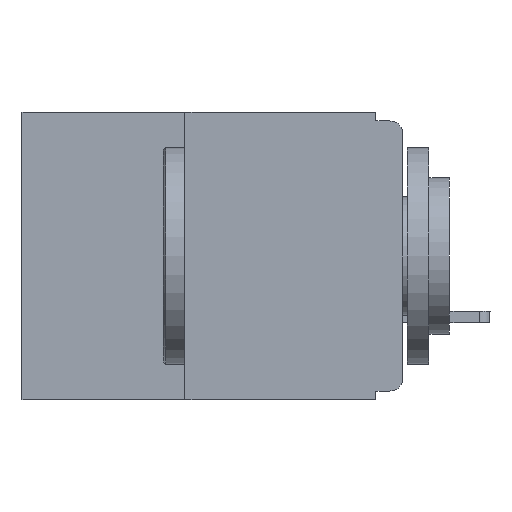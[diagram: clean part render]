
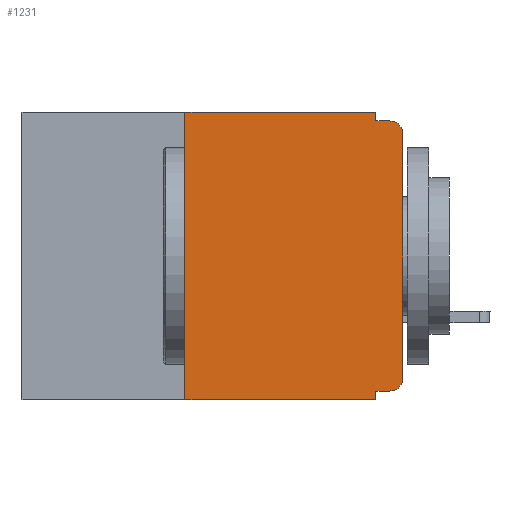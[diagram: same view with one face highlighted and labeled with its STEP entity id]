
A CAD part, left-side view. The second image highlights one B-rep face of the part: STEP entity #1231.
In plain terms, the highlighted planar face has unit normal (-1, 0, 0).
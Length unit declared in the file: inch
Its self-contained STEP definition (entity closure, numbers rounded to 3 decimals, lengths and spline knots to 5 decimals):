
#400 = CARTESIAN_POINT ( 'NONE',  ( 0., 0.015, -0.025 ) ) ;
#555 = CARTESIAN_POINT ( 'NONE',  ( 0., 0.25, -0.33 ) ) ;
#759 = CARTESIAN_POINT ( 'NONE',  ( 0., 0.031, -0.32 ) ) ;
#765 = CARTESIAN_POINT ( 'NONE',  ( 0., 0.25, -0.33 ) ) ;
#837 = AXIS2_PLACEMENT_3D ( 'NONE', #400, #8403, #2529 ) ;
#1047 = CARTESIAN_POINT ( 'NONE',  ( 0., 0.25, 0. ) ) ;
#1231 = ADVANCED_FACE ( 'NONE', ( #4734 ), #10816, .F. ) ;
#1257 = ORIENTED_EDGE ( 'NONE', *, *, #12819, .T. ) ;
#1426 = VERTEX_POINT ( 'NONE', #13756 ) ;
#1463 = LINE ( 'NONE', #3609, #4878 ) ;
#1474 = EDGE_CURVE ( 'NONE', #14251, #2308, #5824, .T. ) ;
#1595 = DIRECTION ( 'NONE',  ( 0., 1., 0. ) ) ;
#1704 = ORIENTED_EDGE ( 'NONE', *, *, #1474, .T. ) ;
#1735 = CARTESIAN_POINT ( 'NONE',  ( 0., 0., -0.01 ) ) ;
#1940 = EDGE_CURVE ( 'NONE', #13731, #7033, #12587, .T. ) ;
#2224 = CARTESIAN_POINT ( 'NONE',  ( 0., 0.015, -0.01 ) ) ;
#2284 = EDGE_CURVE ( 'NONE', #1426, #12051, #12751, .T. ) ;
#2308 = VERTEX_POINT ( 'NONE', #3808 ) ;
#2529 = DIRECTION ( 'NONE',  ( 0., 0., -1. ) ) ;
#2560 = ORIENTED_EDGE ( 'NONE', *, *, #7017, .F. ) ;
#2959 = VECTOR ( 'NONE', #10893, 39.37008 ) ;
#3289 = ORIENTED_EDGE ( 'NONE', *, *, #1940, .F. ) ;
#3340 = AXIS2_PLACEMENT_3D ( 'NONE', #14226, #7189, #14316 ) ;
#3463 = EDGE_CURVE ( 'NONE', #14881, #12051, #5784, .T. ) ;
#3609 = CARTESIAN_POINT ( 'NONE',  ( 0., 0., 0. ) ) ;
#3663 = DIRECTION ( 'NONE',  ( 0., 0., 1. ) ) ;
#3808 = CARTESIAN_POINT ( 'NONE',  ( 0., 0., -0.305 ) ) ;
#3840 = ORIENTED_EDGE ( 'NONE', *, *, #8504, .T. ) ;
#4064 = EDGE_CURVE ( 'NONE', #6564, #12901, #7020, .T. ) ;
#4211 = CARTESIAN_POINT ( 'NONE',  ( 0., 0.437, -0.33 ) ) ;
#4337 = CARTESIAN_POINT ( 'NONE',  ( 0., 0.031, 0. ) ) ;
#4423 = CARTESIAN_POINT ( 'NONE',  ( 0., 0.031, -0.33 ) ) ;
#4428 = ORIENTED_EDGE ( 'NONE', *, *, #13892, .F. ) ;
#4734 = FACE_OUTER_BOUND ( 'NONE', #10722, .T. ) ;
#4878 = VECTOR ( 'NONE', #3663, 39.37008 ) ;
#5418 = VECTOR ( 'NONE', #10131, 39.37008 ) ;
#5421 = DIRECTION ( 'NONE',  ( 0., -1., 0. ) ) ;
#5551 = CARTESIAN_POINT ( 'NONE',  ( 0., 0.015, -0.305 ) ) ;
#5646 = CARTESIAN_POINT ( 'NONE',  ( 0., 0.437, 0. ) ) ;
#5756 = LINE ( 'NONE', #5646, #6821 ) ;
#5784 = LINE ( 'NONE', #1735, #7935 ) ;
#5824 = CIRCLE ( 'NONE', #11111, 0.015 ) ;
#6564 = VERTEX_POINT ( 'NONE', #759 ) ;
#6794 = CARTESIAN_POINT ( 'NONE',  ( 0., 0.031, 0. ) ) ;
#6795 = DIRECTION ( 'NONE',  ( 0., -1., 0. ) ) ;
#6821 = VECTOR ( 'NONE', #6795, 39.37008 ) ;
#7017 = EDGE_CURVE ( 'NONE', #8080, #14881, #10068, .T. ) ;
#7020 = LINE ( 'NONE', #4423, #5418 ) ;
#7033 = VERTEX_POINT ( 'NONE', #1047 ) ;
#7097 = EDGE_CURVE ( 'NONE', #14251, #6564, #8948, .T. ) ;
#7189 = DIRECTION ( 'NONE',  ( 1., 0., 0. ) ) ;
#7916 = DIRECTION ( 'NONE',  ( 0., 0., -1. ) ) ;
#7935 = VECTOR ( 'NONE', #10973, 39.37008 ) ;
#8024 = ORIENTED_EDGE ( 'NONE', *, *, #7097, .F. ) ;
#8080 = VERTEX_POINT ( 'NONE', #6794 ) ;
#8403 = DIRECTION ( 'NONE',  ( -1., 0., 0. ) ) ;
#8426 = ORIENTED_EDGE ( 'NONE', *, *, #2284, .T. ) ;
#8504 = EDGE_CURVE ( 'NONE', #13731, #12901, #14131, .T. ) ;
#8948 = LINE ( 'NONE', #12123, #11563 ) ;
#9045 = DIRECTION ( 'NONE',  ( -1., 0., 0. ) ) ;
#9204 = ORIENTED_EDGE ( 'NONE', *, *, #4064, .F. ) ;
#10068 = LINE ( 'NONE', #4337, #11917 ) ;
#10131 = DIRECTION ( 'NONE',  ( 0., 0., -1. ) ) ;
#10722 = EDGE_LOOP ( 'NONE', ( #1257, #8426, #14036, #2560, #4428, #3289, #3840, #9204, #8024, #1704 ) ) ;
#10816 = PLANE ( 'NONE',  #3340 ) ;
#10893 = DIRECTION ( 'NONE',  ( 0., 0., 1. ) ) ;
#10973 = DIRECTION ( 'NONE',  ( 0., -1., 0. ) ) ;
#11026 = VECTOR ( 'NONE', #5421, 39.37008 ) ;
#11111 = AXIS2_PLACEMENT_3D ( 'NONE', #5551, #9045, #11214 ) ;
#11214 = DIRECTION ( 'NONE',  ( 0., 0., -1. ) ) ;
#11563 = VECTOR ( 'NONE', #1595, 39.37008 ) ;
#11917 = VECTOR ( 'NONE', #7916, 39.37008 ) ;
#12051 = VERTEX_POINT ( 'NONE', #2224 ) ;
#12123 = CARTESIAN_POINT ( 'NONE',  ( 0., 0., -0.32 ) ) ;
#12587 = LINE ( 'NONE', #555, #2959 ) ;
#12751 = CIRCLE ( 'NONE', #837, 0.015 ) ;
#12819 = EDGE_CURVE ( 'NONE', #2308, #1426, #1463, .T. ) ;
#12901 = VERTEX_POINT ( 'NONE', #13163 ) ;
#13163 = CARTESIAN_POINT ( 'NONE',  ( 0., 0.031, -0.33 ) ) ;
#13332 = CARTESIAN_POINT ( 'NONE',  ( 0., 0.031, -0.01 ) ) ;
#13731 = VERTEX_POINT ( 'NONE', #765 ) ;
#13756 = CARTESIAN_POINT ( 'NONE',  ( 0., 0., -0.025 ) ) ;
#13892 = EDGE_CURVE ( 'NONE', #7033, #8080, #5756, .T. ) ;
#14036 = ORIENTED_EDGE ( 'NONE', *, *, #3463, .F. ) ;
#14131 = LINE ( 'NONE', #4211, #11026 ) ;
#14226 = CARTESIAN_POINT ( 'NONE',  ( 0., 0.437, 0. ) ) ;
#14251 = VERTEX_POINT ( 'NONE', #14735 ) ;
#14316 = DIRECTION ( 'NONE',  ( 0., 0., -1. ) ) ;
#14735 = CARTESIAN_POINT ( 'NONE',  ( 0., 0.015, -0.32 ) ) ;
#14881 = VERTEX_POINT ( 'NONE', #13332 ) ;
